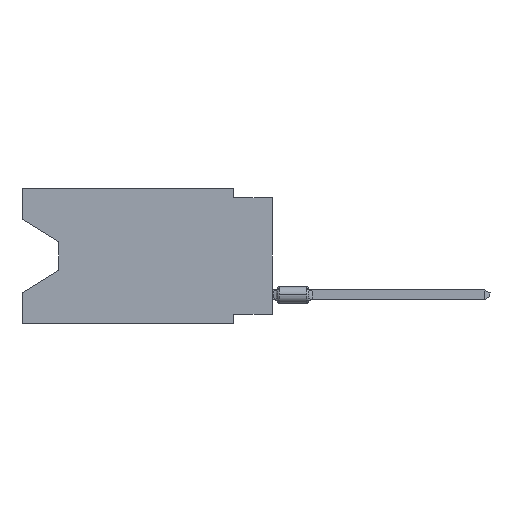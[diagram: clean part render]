
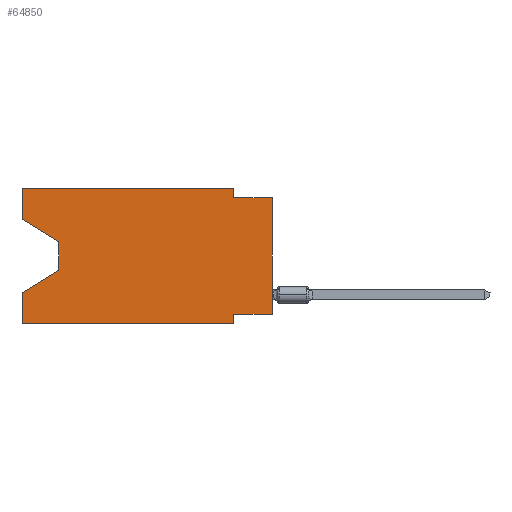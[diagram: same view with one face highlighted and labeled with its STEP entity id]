
A CAD part, left-side view. The second image highlights one B-rep face of the part: STEP entity #64850.
In plain terms, the highlighted planar face has unit normal (-1, 0, 0).
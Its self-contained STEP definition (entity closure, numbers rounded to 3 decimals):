
#149 = DIRECTION ( 'NONE',  ( 0., 0., -1. ) ) ;
#1321 = EDGE_CURVE ( 'NONE', #58611, #40737, #82000, .T. ) ;
#1787 = VERTEX_POINT ( 'NONE', #89565 ) ;
#2759 = EDGE_CURVE ( 'NONE', #12777, #29650, #78102, .T. ) ;
#2886 = ORIENTED_EDGE ( 'NONE', *, *, #42377, .F. ) ;
#4095 = LINE ( 'NONE', #33430, #30391 ) ;
#5477 = ORIENTED_EDGE ( 'NONE', *, *, #38747, .T. ) ;
#5865 = DIRECTION ( 'NONE',  ( 0., 1., 0. ) ) ;
#5904 = CARTESIAN_POINT ( 'NONE',  ( 0., 16.383, 0. ) ) ;
#6421 = LINE ( 'NONE', #41078, #56599 ) ;
#8091 = CARTESIAN_POINT ( 'NONE',  ( 0., 2.54, 0. ) ) ;
#9360 = LINE ( 'NONE', #17516, #21307 ) ;
#9722 = VERTEX_POINT ( 'NONE', #64470 ) ;
#9800 = CARTESIAN_POINT ( 'NONE',  ( 0., 13.97, -5.385 ) ) ;
#10201 = VERTEX_POINT ( 'NONE', #59870 ) ;
#10213 = VERTEX_POINT ( 'NONE', #9800 ) ;
#10246 = ORIENTED_EDGE ( 'NONE', *, *, #40133, .F. ) ;
#12179 = DIRECTION ( 'NONE',  ( 0., 0., -1. ) ) ;
#12777 = VERTEX_POINT ( 'NONE', #41173 ) ;
#12943 = ORIENTED_EDGE ( 'NONE', *, *, #67476, .T. ) ;
#13059 = LINE ( 'NONE', #57331, #83502 ) ;
#17516 = CARTESIAN_POINT ( 'NONE',  ( 0., 0., -0.635 ) ) ;
#17701 = VERTEX_POINT ( 'NONE', #64613 ) ;
#18496 = ORIENTED_EDGE ( 'NONE', *, *, #19516, .T. ) ;
#18750 = AXIS2_PLACEMENT_3D ( 'NONE', #5904, #93457, #92508 ) ;
#19208 = VECTOR ( 'NONE', #55007, 1000. ) ;
#19516 = EDGE_CURVE ( 'NONE', #92544, #29650, #87658, .T. ) ;
#19611 = DIRECTION ( 'NONE',  ( 0., 0.855, -0.519 ) ) ;
#19867 = DIRECTION ( 'NONE',  ( 0., 0., 1. ) ) ;
#20258 = ORIENTED_EDGE ( 'NONE', *, *, #92501, .F. ) ;
#20571 = LINE ( 'NONE', #78327, #84641 ) ;
#20828 = CARTESIAN_POINT ( 'NONE',  ( 0., 16.383, -8.89 ) ) ;
#21307 = VECTOR ( 'NONE', #40137, 1000. ) ;
#21666 = CARTESIAN_POINT ( 'NONE',  ( 0., 0., -8.255 ) ) ;
#25663 = LINE ( 'NONE', #48727, #19208 ) ;
#25684 = CARTESIAN_POINT ( 'NONE',  ( 0., 2.54, -8.89 ) ) ;
#27648 = CARTESIAN_POINT ( 'NONE',  ( 0., 2.54, -8.89 ) ) ;
#28736 = VECTOR ( 'NONE', #71825, 1000. ) ;
#28997 = CARTESIAN_POINT ( 'NONE',  ( 0., 16.383, 0. ) ) ;
#29650 = VERTEX_POINT ( 'NONE', #27648 ) ;
#30391 = VECTOR ( 'NONE', #62770, 1000. ) ;
#30991 = CARTESIAN_POINT ( 'NONE',  ( 0., 0., 0. ) ) ;
#33430 = CARTESIAN_POINT ( 'NONE',  ( 0., 13.97, -3.505 ) ) ;
#33810 = PLANE ( 'NONE',  #18750 ) ;
#36204 = LINE ( 'NONE', #65565, #81744 ) ;
#38747 = EDGE_CURVE ( 'NONE', #10213, #9722, #20571, .T. ) ;
#39336 = VERTEX_POINT ( 'NONE', #66744 ) ;
#40133 = EDGE_CURVE ( 'NONE', #44633, #39336, #36204, .T. ) ;
#40137 = DIRECTION ( 'NONE',  ( 0., -1., 0. ) ) ;
#40737 = VERTEX_POINT ( 'NONE', #83896 ) ;
#41078 = CARTESIAN_POINT ( 'NONE',  ( 0., 16.383, 0. ) ) ;
#41173 = CARTESIAN_POINT ( 'NONE',  ( 0., 2.54, -8.255 ) ) ;
#42377 = EDGE_CURVE ( 'NONE', #10201, #44633, #53026, .T. ) ;
#44633 = VERTEX_POINT ( 'NONE', #8091 ) ;
#46274 = CARTESIAN_POINT ( 'NONE',  ( 0., 16.383, 0. ) ) ;
#46553 = EDGE_CURVE ( 'NONE', #17701, #10213, #4095, .T. ) ;
#47903 = EDGE_CURVE ( 'NONE', #39336, #40737, #9360, .T. ) ;
#48727 = CARTESIAN_POINT ( 'NONE',  ( 0., 16.383, -2.038 ) ) ;
#49164 = DIRECTION ( 'NONE',  ( 0., -1., 0. ) ) ;
#49873 = ORIENTED_EDGE ( 'NONE', *, *, #47903, .F. ) ;
#50168 = VECTOR ( 'NONE', #12179, 1000. ) ;
#53026 = LINE ( 'NONE', #46274, #68195 ) ;
#53792 = ORIENTED_EDGE ( 'NONE', *, *, #59959, .F. ) ;
#55007 = DIRECTION ( 'NONE',  ( 0., -0.855, -0.519 ) ) ;
#56397 = CARTESIAN_POINT ( 'NONE',  ( 0., 16.383, -8.89 ) ) ;
#56599 = VECTOR ( 'NONE', #19867, 1000. ) ;
#57331 = CARTESIAN_POINT ( 'NONE',  ( 0., 0., -8.255 ) ) ;
#58611 = VERTEX_POINT ( 'NONE', #21666 ) ;
#59870 = CARTESIAN_POINT ( 'NONE',  ( 0., 16.383, 0. ) ) ;
#59959 = EDGE_CURVE ( 'NONE', #58611, #12777, #13059, .T. ) ;
#62519 = ORIENTED_EDGE ( 'NONE', *, *, #90899, .F. ) ;
#62770 = DIRECTION ( 'NONE',  ( 0., 0., -1. ) ) ;
#64161 = ORIENTED_EDGE ( 'NONE', *, *, #2759, .F. ) ;
#64470 = CARTESIAN_POINT ( 'NONE',  ( 0., 16.383, -6.852 ) ) ;
#64613 = CARTESIAN_POINT ( 'NONE',  ( 0., 13.97, -3.505 ) ) ;
#64850 = ADVANCED_FACE ( 'NONE', ( #65061 ), #33810, .F. ) ;
#65061 = FACE_OUTER_BOUND ( 'NONE', #93743, .T. ) ;
#65565 = CARTESIAN_POINT ( 'NONE',  ( 0., 2.54, 0. ) ) ;
#66744 = CARTESIAN_POINT ( 'NONE',  ( 0., 2.54, -0.635 ) ) ;
#67476 = EDGE_CURVE ( 'NONE', #1787, #17701, #25663, .T. ) ;
#68195 = VECTOR ( 'NONE', #76087, 1000. ) ;
#71825 = DIRECTION ( 'NONE',  ( 0., 0., 1. ) ) ;
#73059 = VECTOR ( 'NONE', #49164, 1000. ) ;
#74467 = ORIENTED_EDGE ( 'NONE', *, *, #46553, .T. ) ;
#76087 = DIRECTION ( 'NONE',  ( 0., -1., 0. ) ) ;
#78102 = LINE ( 'NONE', #25684, #50168 ) ;
#78327 = CARTESIAN_POINT ( 'NONE',  ( 0., 13.97, -5.385 ) ) ;
#81744 = VECTOR ( 'NONE', #149, 1000. ) ;
#82000 = LINE ( 'NONE', #30991, #86858 ) ;
#83423 = DIRECTION ( 'NONE',  ( 0., 0., 1. ) ) ;
#83502 = VECTOR ( 'NONE', #5865, 1000. ) ;
#83896 = CARTESIAN_POINT ( 'NONE',  ( 0., 0., -0.635 ) ) ;
#84641 = VECTOR ( 'NONE', #19611, 1000. ) ;
#86858 = VECTOR ( 'NONE', #83423, 1000. ) ;
#87658 = LINE ( 'NONE', #56397, #73059 ) ;
#87695 = LINE ( 'NONE', #28997, #28736 ) ;
#88348 = ORIENTED_EDGE ( 'NONE', *, *, #1321, .T. ) ;
#89565 = CARTESIAN_POINT ( 'NONE',  ( 0., 16.383, -2.038 ) ) ;
#90899 = EDGE_CURVE ( 'NONE', #1787, #10201, #87695, .T. ) ;
#92501 = EDGE_CURVE ( 'NONE', #92544, #9722, #6421, .T. ) ;
#92508 = DIRECTION ( 'NONE',  ( 0., 0., -1. ) ) ;
#92544 = VERTEX_POINT ( 'NONE', #20828 ) ;
#93457 = DIRECTION ( 'NONE',  ( 1., 0., 0. ) ) ;
#93743 = EDGE_LOOP ( 'NONE', ( #12943, #74467, #5477, #20258, #18496, #64161, #53792, #88348, #49873, #10246, #2886, #62519 ) ) ;
